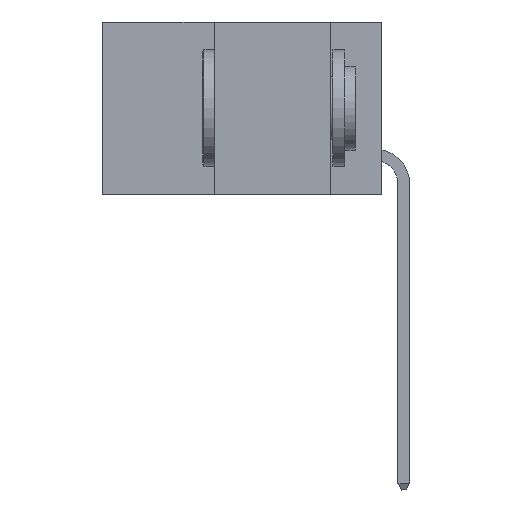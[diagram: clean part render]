
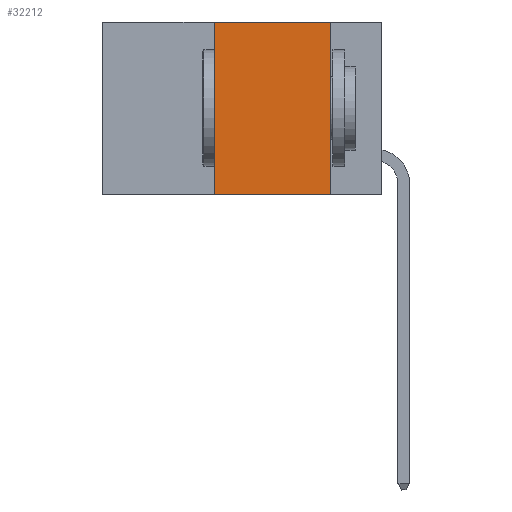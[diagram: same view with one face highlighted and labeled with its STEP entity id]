
A CAD part, left-side view. The second image highlights one B-rep face of the part: STEP entity #32212.
In plain terms, the highlighted planar face has unit normal (-1, 0, 0).
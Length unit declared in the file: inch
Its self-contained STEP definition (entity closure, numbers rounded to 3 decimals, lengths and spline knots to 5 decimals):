
#2132 = EDGE_CURVE ( 'NONE', #11093, #6080, #41555, .T. ) ;
#2739 = PLANE ( 'NONE',  #41669 ) ;
#5075 = CARTESIAN_POINT ( 'NONE',  ( 0., 0.11, -0.37 ) ) ;
#6080 = VERTEX_POINT ( 'NONE', #13319 ) ;
#6536 = VECTOR ( 'NONE', #34114, 39.37008 ) ;
#6886 = EDGE_CURVE ( 'NONE', #10196, #11093, #26990, .T. ) ;
#9314 = DIRECTION ( 'NONE',  ( 0., 0., -1. ) ) ;
#9757 = DIRECTION ( 'NONE',  ( 0., -1., 0. ) ) ;
#10196 = VERTEX_POINT ( 'NONE', #14838 ) ;
#10503 = DIRECTION ( 'NONE',  ( 0., 0., -1. ) ) ;
#11093 = VERTEX_POINT ( 'NONE', #35804 ) ;
#11418 = VECTOR ( 'NONE', #10503, 39.37008 ) ;
#12052 = CARTESIAN_POINT ( 'NONE',  ( 0., 0.6, 0. ) ) ;
#13319 = CARTESIAN_POINT ( 'NONE',  ( 0., 0.11, 0. ) ) ;
#14253 = CARTESIAN_POINT ( 'NONE',  ( 0., 0.36, 0. ) ) ;
#14838 = CARTESIAN_POINT ( 'NONE',  ( 0., 0.36, -0.37 ) ) ;
#15582 = EDGE_LOOP ( 'NONE', ( #29084, #40320, #31481, #25967 ) ) ;
#19839 = CARTESIAN_POINT ( 'NONE',  ( 0., 0.6, 0. ) ) ;
#20448 = VERTEX_POINT ( 'NONE', #5075 ) ;
#24310 = FACE_OUTER_BOUND ( 'NONE', #15582, .T. ) ;
#24591 = VECTOR ( 'NONE', #9757, 39.37008 ) ;
#25967 = ORIENTED_EDGE ( 'NONE', *, *, #34631, .T. ) ;
#26073 = CARTESIAN_POINT ( 'NONE',  ( 0., 0.6, -0.37 ) ) ;
#26990 = LINE ( 'NONE', #14253, #6536 ) ;
#27592 = EDGE_CURVE ( 'NONE', #6080, #20448, #28802, .T. ) ;
#28802 = LINE ( 'NONE', #36404, #11418 ) ;
#29084 = ORIENTED_EDGE ( 'NONE', *, *, #27592, .F. ) ;
#29097 = DIRECTION ( 'NONE',  ( 0., -1., 0. ) ) ;
#31481 = ORIENTED_EDGE ( 'NONE', *, *, #6886, .F. ) ;
#31892 = DIRECTION ( 'NONE',  ( 1., 0., 0. ) ) ;
#32212 = ADVANCED_FACE ( 'NONE', ( #24310 ), #2739, .F. ) ;
#34114 = DIRECTION ( 'NONE',  ( 0., 0., 1. ) ) ;
#34631 = EDGE_CURVE ( 'NONE', #10196, #20448, #36370, .T. ) ;
#35804 = CARTESIAN_POINT ( 'NONE',  ( 0., 0.36, 0. ) ) ;
#35946 = VECTOR ( 'NONE', #29097, 39.37008 ) ;
#36370 = LINE ( 'NONE', #26073, #24591 ) ;
#36404 = CARTESIAN_POINT ( 'NONE',  ( 0., 0.11, 0. ) ) ;
#40320 = ORIENTED_EDGE ( 'NONE', *, *, #2132, .F. ) ;
#41555 = LINE ( 'NONE', #19839, #35946 ) ;
#41669 = AXIS2_PLACEMENT_3D ( 'NONE', #12052, #31892, #9314 ) ;
